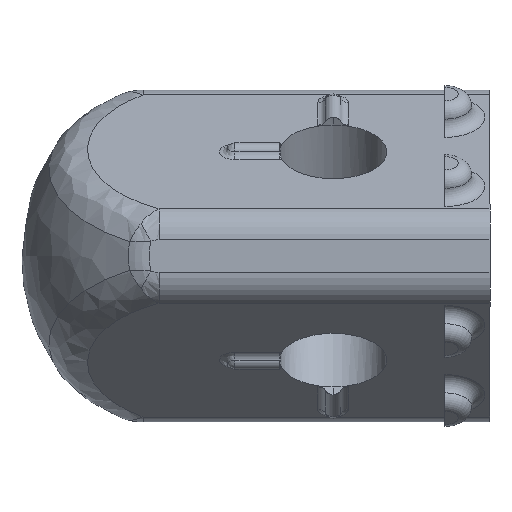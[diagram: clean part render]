
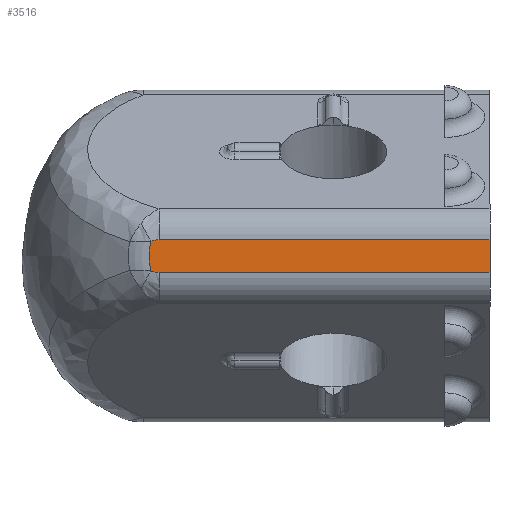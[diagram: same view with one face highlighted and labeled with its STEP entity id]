
A CAD part, left-side view. The second image highlights one B-rep face of the part: STEP entity #3516.
In plain terms, the highlighted planar face has unit normal (-1, 0, 0).
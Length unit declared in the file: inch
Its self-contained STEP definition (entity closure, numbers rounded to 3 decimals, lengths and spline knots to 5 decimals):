
#51 = CARTESIAN_POINT ( 'NONE',  ( 3.96945, -5.16612, 0.10908 ) ) ;
#254 = VERTEX_POINT ( 'NONE', #4510 ) ;
#275 = DIRECTION ( 'NONE',  ( 0., 0., 1. ) ) ;
#365 = CARTESIAN_POINT ( 'NONE',  ( 3.96945, -10.58161, 0.10724 ) ) ;
#404 = DIRECTION ( 'NONE',  ( 1., 0., 0. ) ) ;
#444 = EDGE_CURVE ( 'NONE', #4390, #254, #2187, .T. ) ;
#445 = CARTESIAN_POINT ( 'NONE',  ( 3.96945, -5.15133, 0.11413 ) ) ;
#449 = CARTESIAN_POINT ( 'NONE',  ( 3.96945, -5.15704, 0.11153 ) ) ;
#468 = B_SPLINE_CURVE_WITH_KNOTS ( 'NONE', 3,
 ( #1586, #3804, #2346, #51, #2731, #449, #3115, #843 ),
 .UNSPECIFIED., .F., .F.,
 ( 4, 2, 2, 4 ),
 ( 0., 0.5, 0.75, 1. ),
 .UNSPECIFIED. ) ;
#727 = CARTESIAN_POINT ( 'NONE',  ( 3.96945, -10.58161, 0.25082 ) ) ;
#788 = CARTESIAN_POINT ( 'NONE',  ( 3.96945, -5.16304, 0.24832 ) ) ;
#843 = CARTESIAN_POINT ( 'NONE',  ( 3.96945, -5.15133, 0.11413 ) ) ;
#1156 = EDGE_LOOP ( 'NONE', ( #2748, #2653, #1326, #2632, #1515, #1521 ) ) ;
#1161 = CARTESIAN_POINT ( 'NONE',  ( 3.96945, -10.58161, 0.91 ) ) ;
#1167 = CARTESIAN_POINT ( 'NONE',  ( 3.96945, -5.17536, 0.25047 ) ) ;
#1226 = CARTESIAN_POINT ( 'NONE',  ( 3.96945, -5.15133, 0.24393 ) ) ;
#1295 = EDGE_CURVE ( 'NONE', #4438, #4390, #468, .T. ) ;
#1326 = ORIENTED_EDGE ( 'NONE', *, *, #3087, .F. ) ;
#1477 = VECTOR ( 'NONE', #4077, 39.37008 ) ;
#1484 = DIRECTION ( 'NONE',  ( 0., 1., 0. ) ) ;
#1515 = ORIENTED_EDGE ( 'NONE', *, *, #1295, .F. ) ;
#1521 = ORIENTED_EDGE ( 'NONE', *, *, #2030, .F. ) ;
#1544 = CARTESIAN_POINT ( 'NONE',  ( 3.96945, -5.18785, 0.25082 ) ) ;
#1586 = CARTESIAN_POINT ( 'NONE',  ( 3.96945, -5.18785, 0.10724 ) ) ;
#1597 = LINE ( 'NONE', #727, #1477 ) ;
#2030 = EDGE_CURVE ( 'NONE', #2636, #4438, #3314, .T. ) ;
#2074 = CARTESIAN_POINT ( 'NONE',  ( 3.96945, -6.64698, 0.25082 ) ) ;
#2187 =( BOUNDED_CURVE ( )  B_SPLINE_CURVE ( 3, ( #445, #3813, #3474, #1226 ),
 .UNSPECIFIED., .F., .T. ) 
 B_SPLINE_CURVE_WITH_KNOTS ( ( 4, 4 ),
 ( 0., 1. ),
 .UNSPECIFIED. ) 
 CURVE ( )  GEOMETRIC_REPRESENTATION_ITEM ( )  RATIONAL_B_SPLINE_CURVE ( ( 1., 0.986, 0.986, 1. ) ) 
 REPRESENTATION_ITEM ( '' )  );
#2255 = CARTESIAN_POINT ( 'NONE',  ( 3.96945, -5.18785, 0.10724 ) ) ;
#2346 = CARTESIAN_POINT ( 'NONE',  ( 3.96945, -5.17536, 0.1076 ) ) ;
#2364 = B_SPLINE_CURVE_WITH_KNOTS ( 'NONE', 3,
 ( #3030, #3049, #3067, #788, #3413, #1167, #3769, #1544 ),
 .UNSPECIFIED., .F., .F.,
 ( 4, 2, 2, 4 ),
 ( 0., 0.25, 0.5, 1. ),
 .UNSPECIFIED. ) ;
#2473 = VERTEX_POINT ( 'NONE', #4596 ) ;
#2574 = CARTESIAN_POINT ( 'NONE',  ( 3.96945, -6.64698, 37.83559 ) ) ;
#2613 = CARTESIAN_POINT ( 'NONE',  ( 3.96945, -5.15133, 0.11413 ) ) ;
#2632 = ORIENTED_EDGE ( 'NONE', *, *, #444, .F. ) ;
#2636 = VERTEX_POINT ( 'NONE', #4019 ) ;
#2653 = ORIENTED_EDGE ( 'NONE', *, *, #2718, .F. ) ;
#2718 = EDGE_CURVE ( 'NONE', #2473, #3775, #1597, .T. ) ;
#2731 = CARTESIAN_POINT ( 'NONE',  ( 3.96945, -5.16304, 0.10975 ) ) ;
#2748 = ORIENTED_EDGE ( 'NONE', *, *, #4728, .T. ) ;
#2948 = LINE ( 'NONE', #2574, #4729 ) ;
#3030 = CARTESIAN_POINT ( 'NONE',  ( 3.96945, -5.15133, 0.24393 ) ) ;
#3049 = CARTESIAN_POINT ( 'NONE',  ( 3.96945, -5.15412, 0.24541 ) ) ;
#3067 = CARTESIAN_POINT ( 'NONE',  ( 3.96945, -5.15704, 0.24653 ) ) ;
#3075 = DIRECTION ( 'NONE',  ( 0., 1., 0. ) ) ;
#3087 = EDGE_CURVE ( 'NONE', #254, #2473, #2364, .T. ) ;
#3115 = CARTESIAN_POINT ( 'NONE',  ( 3.96945, -5.15412, 0.11265 ) ) ;
#3314 = LINE ( 'NONE', #365, #3809 ) ;
#3413 = CARTESIAN_POINT ( 'NONE',  ( 3.96945, -5.16612, 0.24898 ) ) ;
#3474 = CARTESIAN_POINT ( 'NONE',  ( 3.96945, -5.1424, 0.20097 ) ) ;
#3516 = ADVANCED_FACE ( 'NONE', ( #3586 ), #4477, .F. ) ;
#3586 = FACE_OUTER_BOUND ( 'NONE', #1156, .T. ) ;
#3769 = CARTESIAN_POINT ( 'NONE',  ( 3.96945, -5.18159, 0.25082 ) ) ;
#3775 = VERTEX_POINT ( 'NONE', #2074 ) ;
#3804 = CARTESIAN_POINT ( 'NONE',  ( 3.96945, -5.18159, 0.10724 ) ) ;
#3809 = VECTOR ( 'NONE', #1484, 39.37008 ) ;
#3813 = CARTESIAN_POINT ( 'NONE',  ( 3.96945, -5.1424, 0.15709 ) ) ;
#4019 = CARTESIAN_POINT ( 'NONE',  ( 3.96945, -6.64698, 0.10724 ) ) ;
#4077 = DIRECTION ( 'NONE',  ( 0., -1., 0. ) ) ;
#4390 = VERTEX_POINT ( 'NONE', #2613 ) ;
#4438 = VERTEX_POINT ( 'NONE', #2255 ) ;
#4477 = PLANE ( 'NONE',  #4798 ) ;
#4510 = CARTESIAN_POINT ( 'NONE',  ( 3.96945, -5.15133, 0.24393 ) ) ;
#4596 = CARTESIAN_POINT ( 'NONE',  ( 3.96945, -5.18785, 0.25082 ) ) ;
#4728 = EDGE_CURVE ( 'NONE', #2636, #3775, #2948, .T. ) ;
#4729 = VECTOR ( 'NONE', #275, 39.37008 ) ;
#4798 = AXIS2_PLACEMENT_3D ( 'NONE', #1161, #404, #3075 ) ;
